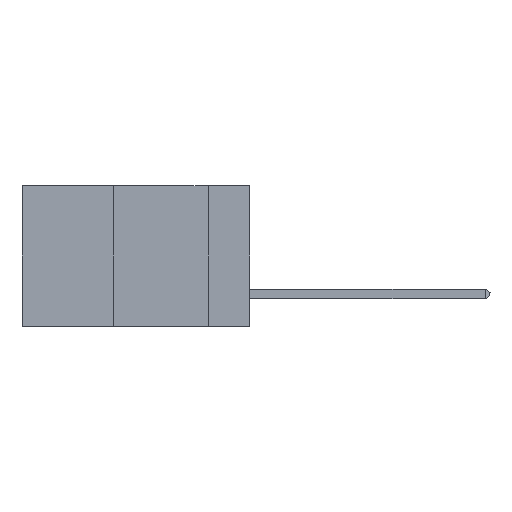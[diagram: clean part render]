
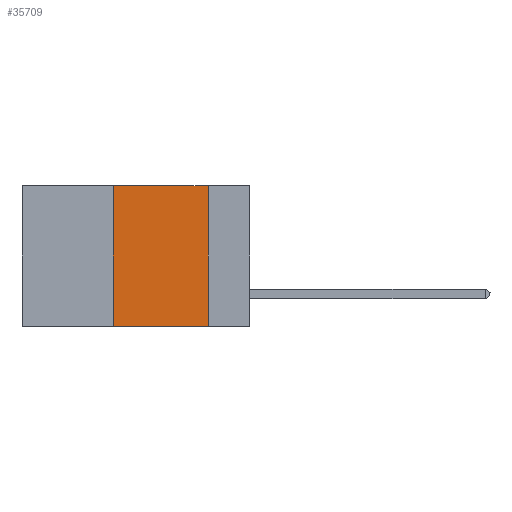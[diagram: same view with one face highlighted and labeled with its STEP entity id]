
A CAD part, left-side view. The second image highlights one B-rep face of the part: STEP entity #35709.
In plain terms, the highlighted planar face has unit normal (-1, 0, 0).
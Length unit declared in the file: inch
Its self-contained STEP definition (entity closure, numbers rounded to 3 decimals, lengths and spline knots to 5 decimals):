
#4456 = EDGE_CURVE ( 'NONE', #42753, #29758, #46517, .T. ) ;
#6682 = EDGE_LOOP ( 'NONE', ( #19044, #20196, #47794, #44774 ) ) ;
#7000 = LINE ( 'NONE', #41752, #15361 ) ;
#9211 = CARTESIAN_POINT ( 'NONE',  ( 0., 0.36, -0.37 ) ) ;
#9227 = CARTESIAN_POINT ( 'NONE',  ( 0., 0.6, -0.37 ) ) ;
#12717 = EDGE_CURVE ( 'NONE', #42753, #28805, #40877, .T. ) ;
#13875 = LINE ( 'NONE', #38760, #36042 ) ;
#14085 = DIRECTION ( 'NONE',  ( 0., 0., -1. ) ) ;
#15361 = VECTOR ( 'NONE', #26445, 39.37008 ) ;
#15768 = DIRECTION ( 'NONE',  ( 0., 0., -1. ) ) ;
#17568 = DIRECTION ( 'NONE',  ( 1., 0., 0. ) ) ;
#19044 = ORIENTED_EDGE ( 'NONE', *, *, #38666, .F. ) ;
#20196 = ORIENTED_EDGE ( 'NONE', *, *, #43314, .F. ) ;
#21573 = DIRECTION ( 'NONE',  ( 0., 0., 1. ) ) ;
#26445 = DIRECTION ( 'NONE',  ( 0., -1., 0. ) ) ;
#28155 = DIRECTION ( 'NONE',  ( 0., -1., 0. ) ) ;
#28805 = VERTEX_POINT ( 'NONE', #47265 ) ;
#29662 = PLANE ( 'NONE',  #29839 ) ;
#29758 = VERTEX_POINT ( 'NONE', #33745 ) ;
#29839 = AXIS2_PLACEMENT_3D ( 'NONE', #37047, #17568, #14085 ) ;
#33671 = CARTESIAN_POINT ( 'NONE',  ( 0., 0.36, 0. ) ) ;
#33697 = VECTOR ( 'NONE', #21573, 39.37008 ) ;
#33745 = CARTESIAN_POINT ( 'NONE',  ( 0., 0.11, -0.37 ) ) ;
#35709 = ADVANCED_FACE ( 'NONE', ( #48890 ), #29662, .F. ) ;
#36042 = VECTOR ( 'NONE', #15768, 39.37008 ) ;
#37047 = CARTESIAN_POINT ( 'NONE',  ( 0., 0.6, 0. ) ) ;
#38666 = EDGE_CURVE ( 'NONE', #43296, #29758, #13875, .T. ) ;
#38760 = CARTESIAN_POINT ( 'NONE',  ( 0., 0.11, 0. ) ) ;
#40877 = LINE ( 'NONE', #33671, #33697 ) ;
#41752 = CARTESIAN_POINT ( 'NONE',  ( 0., 0.6, 0. ) ) ;
#42753 = VERTEX_POINT ( 'NONE', #9211 ) ;
#43296 = VERTEX_POINT ( 'NONE', #48928 ) ;
#43314 = EDGE_CURVE ( 'NONE', #28805, #43296, #7000, .T. ) ;
#44774 = ORIENTED_EDGE ( 'NONE', *, *, #4456, .T. ) ;
#45329 = VECTOR ( 'NONE', #28155, 39.37008 ) ;
#46517 = LINE ( 'NONE', #9227, #45329 ) ;
#47265 = CARTESIAN_POINT ( 'NONE',  ( 0., 0.36, 0. ) ) ;
#47794 = ORIENTED_EDGE ( 'NONE', *, *, #12717, .F. ) ;
#48890 = FACE_OUTER_BOUND ( 'NONE', #6682, .T. ) ;
#48928 = CARTESIAN_POINT ( 'NONE',  ( 0., 0.11, 0. ) ) ;
